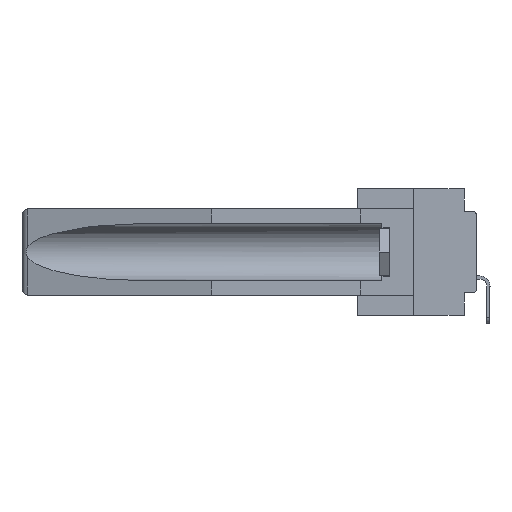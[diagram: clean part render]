
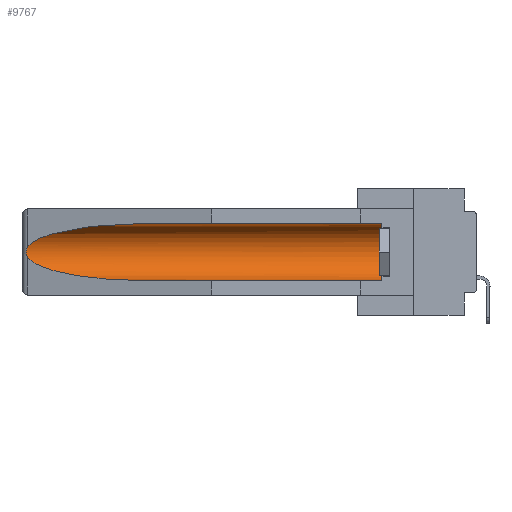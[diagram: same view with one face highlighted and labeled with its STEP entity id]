
A CAD part, left-side view. The second image highlights one B-rep face of the part: STEP entity #9767.
In plain terms, the highlighted cylindrical face has radius 2.857 mm (diameter 5.715 mm), a partial arc.
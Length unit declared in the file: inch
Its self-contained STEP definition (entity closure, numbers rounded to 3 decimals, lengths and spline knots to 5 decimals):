
#852 = EDGE_CURVE ( 'NONE', #5891, #27291, #13449, .T. ) ;
#1799 = EDGE_CURVE ( 'NONE', #29708, #16394, #17500, .T. ) ;
#2033 = EDGE_CURVE ( 'NONE', #16394, #35122, #13963, .T. ) ;
#2076 = CARTESIAN_POINT ( 'NONE',  ( 0.26655, 1.53094, -0.18657 ) ) ;
#2078 = ORIENTED_EDGE ( 'NONE', *, *, #1799, .T. ) ;
#2268 = CARTESIAN_POINT ( 'NONE',  ( 0.26597, 1.5296, -0.19026 ) ) ;
#4119 = CARTESIAN_POINT ( 'NONE',  ( 0.25451, 1.48313, -0.24835 ) ) ;
#4264 = CARTESIAN_POINT ( 'NONE',  ( 0.155, -0.30754, -0.1715 ) ) ;
#4422 = AXIS2_PLACEMENT_3D ( 'NONE', #5161, #22873, #19646 ) ;
#4635 = VECTOR ( 'NONE', #23884, 39.37008 ) ;
#5161 = CARTESIAN_POINT ( 'NONE',  ( 0.155, 0.126, -0.1715 ) ) ;
#5292 = DIRECTION ( 'NONE',  ( 0., 1., 0. ) ) ;
#5477 = CARTESIAN_POINT ( 'NONE',  ( 0.155, 1.07973, -0.059 ) ) ;
#5891 = VERTEX_POINT ( 'NONE', #18228 ) ;
#7279 = DIRECTION ( 'NONE',  ( 0., 1., 0. ) ) ;
#8479 = CARTESIAN_POINT ( 'NONE',  ( 0.26537, 1.52718, -0.14972 ) ) ;
#9183 = CARTESIAN_POINT ( 'NONE',  ( 0.155, 1.07973, -0.284 ) ) ;
#9767 = ADVANCED_FACE ( 'NONE', ( #21771 ), #18935, .F. ) ;
#9776 = LINE ( 'NONE', #32309, #4635 ) ;
#11078 = CARTESIAN_POINT ( 'NONE',  ( 0.26597, 1.52961, -0.15275 ) ) ;
#11704 = VERTEX_POINT ( 'NONE', #15086 ) ;
#12937 = ORIENTED_EDGE ( 'NONE', *, *, #14248, .T. ) ;
#13449 = CIRCLE ( 'NONE', #4422, 0.1125 ) ;
#13760 = CARTESIAN_POINT ( 'NONE',  ( 0.25451, 1.48313, -0.09465 ) ) ;
#13963 =( BOUNDED_CURVE ( )  B_SPLINE_CURVE ( 3, ( #21260, #4119, #33226, #24245 ),
 .UNSPECIFIED., .F., .F. ) 
 B_SPLINE_CURVE_WITH_KNOTS ( ( 4, 4 ),
 ( 0.1948, 1.5708 ),
 .UNSPECIFIED. ) 
 CURVE ( )  GEOMETRIC_REPRESENTATION_ITEM ( )  RATIONAL_B_SPLINE_CURVE ( ( 1., 0.848, 0.848, 1. ) ) 
 REPRESENTATION_ITEM ( '' )  );
#14038 = CARTESIAN_POINT ( 'NONE',  ( 0.26537, 1.52718, -0.19328 ) ) ;
#14248 = EDGE_CURVE ( 'NONE', #11704, #29708, #21686, .T. ) ;
#14284 = EDGE_CURVE ( 'NONE', #27291, #11704, #19225, .T. ) ;
#15086 = CARTESIAN_POINT ( 'NONE',  ( 0.155, 1.07973, -0.059 ) ) ;
#16394 = VERTEX_POINT ( 'NONE', #14038 ) ;
#17500 = B_SPLINE_CURVE_WITH_KNOTS ( 'NONE', 3,
 ( #8479, #11078, #22398, #36435, #31374, #30644, #28179, #2076, #2268, #22581 ),
 .UNSPECIFIED., .F., .F.,
 ( 4, 2, 2, 2, 4 ),
 ( 0., 0.00029, 0.00058, 0.00087, 0.00117 ),
 .UNSPECIFIED. ) ;
#18228 = CARTESIAN_POINT ( 'NONE',  ( 0.155, 0.126, -0.284 ) ) ;
#18935 = CYLINDRICAL_SURFACE ( 'NONE', #25819, 0.1125 ) ;
#18937 = ORIENTED_EDGE ( 'NONE', *, *, #26448, .F. ) ;
#19225 = LINE ( 'NONE', #25606, #33433 ) ;
#19509 = CARTESIAN_POINT ( 'NONE',  ( 0.26537, 1.52718, -0.14972 ) ) ;
#19646 = DIRECTION ( 'NONE',  ( 0., 0., 1. ) ) ;
#21260 = CARTESIAN_POINT ( 'NONE',  ( 0.26537, 1.52718, -0.19328 ) ) ;
#21402 = DIRECTION ( 'NONE',  ( 0., 0., 1. ) ) ;
#21686 =( BOUNDED_CURVE ( )  B_SPLINE_CURVE ( 3, ( #5477, #33666, #13760, #30840 ),
 .UNSPECIFIED., .F., .F. ) 
 B_SPLINE_CURVE_WITH_KNOTS ( ( 4, 4 ),
 ( 4.71239, 6.08839 ),
 .UNSPECIFIED. ) 
 CURVE ( )  GEOMETRIC_REPRESENTATION_ITEM ( )  RATIONAL_B_SPLINE_CURVE ( ( 1., 0.848, 0.848, 1. ) ) 
 REPRESENTATION_ITEM ( '' )  );
#21771 = FACE_OUTER_BOUND ( 'NONE', #22423, .T. ) ;
#22398 = CARTESIAN_POINT ( 'NONE',  ( 0.26654, 1.53092, -0.15636 ) ) ;
#22423 = EDGE_LOOP ( 'NONE', ( #12937, #2078, #35064, #18937, #37067, #34629 ) ) ;
#22581 = CARTESIAN_POINT ( 'NONE',  ( 0.26537, 1.52718, -0.19328 ) ) ;
#22873 = DIRECTION ( 'NONE',  ( 0., -1., 0. ) ) ;
#23884 = DIRECTION ( 'NONE',  ( 0., 1., 0. ) ) ;
#23974 = CARTESIAN_POINT ( 'NONE',  ( 0.155, 0.126, -0.059 ) ) ;
#24245 = CARTESIAN_POINT ( 'NONE',  ( 0.155, 1.07973, -0.284 ) ) ;
#25606 = CARTESIAN_POINT ( 'NONE',  ( 0.155, -0.30754, -0.059 ) ) ;
#25819 = AXIS2_PLACEMENT_3D ( 'NONE', #4264, #7279, #21402 ) ;
#26448 = EDGE_CURVE ( 'NONE', #5891, #35122, #9776, .T. ) ;
#27291 = VERTEX_POINT ( 'NONE', #23974 ) ;
#28179 = CARTESIAN_POINT ( 'NONE',  ( 0.2673, 1.53269, -0.17917 ) ) ;
#29708 = VERTEX_POINT ( 'NONE', #19509 ) ;
#30644 = CARTESIAN_POINT ( 'NONE',  ( 0.2675, 1.53308, -0.17534 ) ) ;
#30840 = CARTESIAN_POINT ( 'NONE',  ( 0.26537, 1.52718, -0.14972 ) ) ;
#31374 = CARTESIAN_POINT ( 'NONE',  ( 0.2675, 1.53308, -0.16763 ) ) ;
#32309 = CARTESIAN_POINT ( 'NONE',  ( 0.155, -0.30754, -0.284 ) ) ;
#33226 = CARTESIAN_POINT ( 'NONE',  ( 0.21114, 1.30732, -0.284 ) ) ;
#33433 = VECTOR ( 'NONE', #5292, 39.37008 ) ;
#33666 = CARTESIAN_POINT ( 'NONE',  ( 0.21114, 1.30732, -0.059 ) ) ;
#34629 = ORIENTED_EDGE ( 'NONE', *, *, #14284, .T. ) ;
#35064 = ORIENTED_EDGE ( 'NONE', *, *, #2033, .T. ) ;
#35122 = VERTEX_POINT ( 'NONE', #9183 ) ;
#36435 = CARTESIAN_POINT ( 'NONE',  ( 0.2673, 1.5327, -0.16383 ) ) ;
#37067 = ORIENTED_EDGE ( 'NONE', *, *, #852, .T. ) ;
